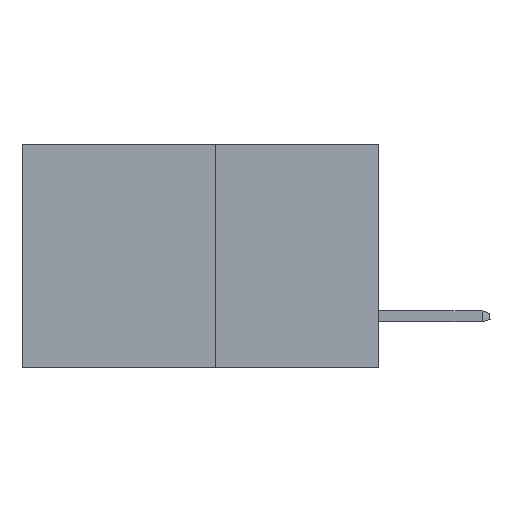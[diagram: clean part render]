
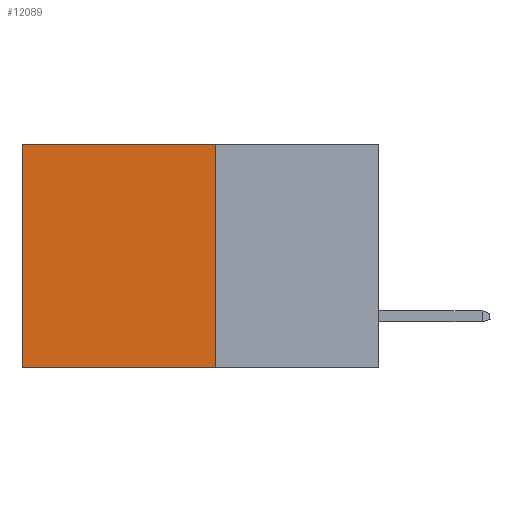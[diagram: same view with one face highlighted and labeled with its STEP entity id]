
A CAD part, left-side view. The second image highlights one B-rep face of the part: STEP entity #12089.
In plain terms, the highlighted planar face has unit normal (-1, 0, 0).
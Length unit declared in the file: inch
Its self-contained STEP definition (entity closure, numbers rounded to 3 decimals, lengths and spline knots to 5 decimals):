
#517 = LINE ( 'NONE', #9588, #14679 ) ;
#648 = CARTESIAN_POINT ( 'NONE',  ( 0.277, 0.27, 0. ) ) ;
#853 = DIRECTION ( 'NONE',  ( 0., 0., -1. ) ) ;
#2455 = ORIENTED_EDGE ( 'NONE', *, *, #15591, .F. ) ;
#3474 = CARTESIAN_POINT ( 'NONE',  ( 0.277, 0.27, -0.37 ) ) ;
#4022 = VECTOR ( 'NONE', #19222, 39.37008 ) ;
#4495 = EDGE_LOOP ( 'NONE', ( #21638, #6803, #2455, #16853 ) ) ;
#4506 = PLANE ( 'NONE',  #17792 ) ;
#4740 = VECTOR ( 'NONE', #14527, 39.37008 ) ;
#5388 = VERTEX_POINT ( 'NONE', #648 ) ;
#5442 = VERTEX_POINT ( 'NONE', #21163 ) ;
#5571 = LINE ( 'NONE', #17762, #11086 ) ;
#5972 = EDGE_CURVE ( 'NONE', #5388, #5442, #9630, .T. ) ;
#6033 = FACE_OUTER_BOUND ( 'NONE', #4495, .T. ) ;
#6803 = ORIENTED_EDGE ( 'NONE', *, *, #21012, .F. ) ;
#8302 = CARTESIAN_POINT ( 'NONE',  ( 0.277, 0.27, -0.37 ) ) ;
#9588 = CARTESIAN_POINT ( 'NONE',  ( 0.277, 0.59, -0.37 ) ) ;
#9630 = LINE ( 'NONE', #19368, #4022 ) ;
#10798 = EDGE_CURVE ( 'NONE', #5442, #17899, #517, .T. ) ;
#11086 = VECTOR ( 'NONE', #15895, 39.37008 ) ;
#11403 = DIRECTION ( 'NONE',  ( 0., 0., -1. ) ) ;
#11971 = DIRECTION ( 'NONE',  ( 1., 0., 0. ) ) ;
#12089 = ADVANCED_FACE ( 'NONE', ( #6033 ), #4506, .F. ) ;
#14527 = DIRECTION ( 'NONE',  ( 0., 0., -1. ) ) ;
#14679 = VECTOR ( 'NONE', #11403, 39.37008 ) ;
#15591 = EDGE_CURVE ( 'NONE', #5388, #20950, #20632, .T. ) ;
#15895 = DIRECTION ( 'NONE',  ( 0., 1., 0. ) ) ;
#16853 = ORIENTED_EDGE ( 'NONE', *, *, #5972, .T. ) ;
#17762 = CARTESIAN_POINT ( 'NONE',  ( 0.277, 0.27, -0.37 ) ) ;
#17792 = AXIS2_PLACEMENT_3D ( 'NONE', #8302, #11971, #853 ) ;
#17899 = VERTEX_POINT ( 'NONE', #22740 ) ;
#19222 = DIRECTION ( 'NONE',  ( 0., 1., 0. ) ) ;
#19368 = CARTESIAN_POINT ( 'NONE',  ( 0.277, 0.27, 0. ) ) ;
#19495 = CARTESIAN_POINT ( 'NONE',  ( 0.277, 0.27, -0.37 ) ) ;
#20632 = LINE ( 'NONE', #3474, #4740 ) ;
#20950 = VERTEX_POINT ( 'NONE', #19495 ) ;
#21012 = EDGE_CURVE ( 'NONE', #20950, #17899, #5571, .T. ) ;
#21163 = CARTESIAN_POINT ( 'NONE',  ( 0.277, 0.59, 0. ) ) ;
#21638 = ORIENTED_EDGE ( 'NONE', *, *, #10798, .T. ) ;
#22740 = CARTESIAN_POINT ( 'NONE',  ( 0.277, 0.59, -0.37 ) ) ;
